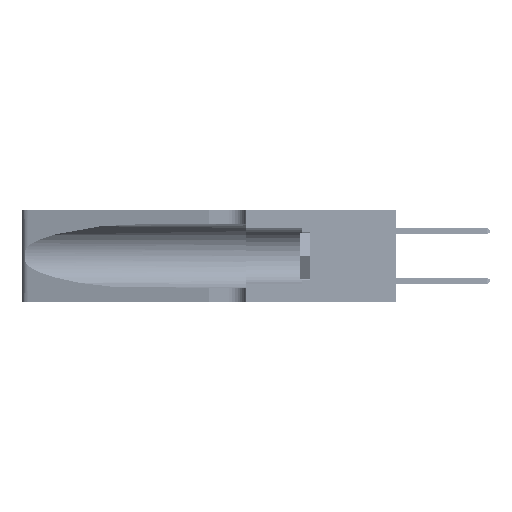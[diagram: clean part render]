
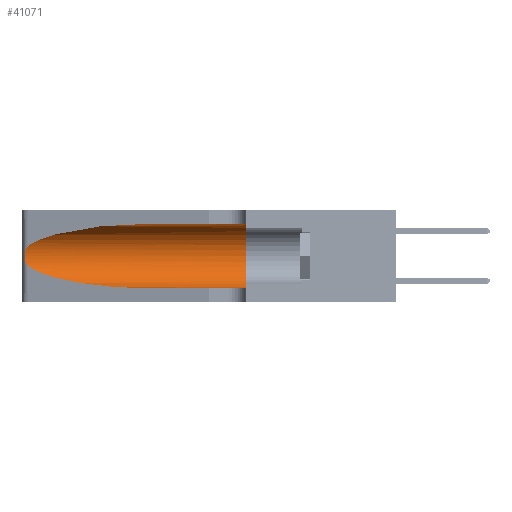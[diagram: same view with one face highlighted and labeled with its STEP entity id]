
A CAD part, left-side view. The second image highlights one B-rep face of the part: STEP entity #41071.
In plain terms, the highlighted cylindrical face has radius 3.308 mm (diameter 6.617 mm), a partial arc.
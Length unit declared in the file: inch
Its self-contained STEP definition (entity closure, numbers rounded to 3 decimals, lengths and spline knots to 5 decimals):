
#475 = CARTESIAN_POINT ( 'NONE',  ( 0.26075, 1.23896, 0.178 ) ) ;
#2468 = ORIENTED_EDGE ( 'NONE', *, *, #50630, .T. ) ;
#2620 = VERTEX_POINT ( 'NONE', #48003 ) ;
#3009 = VERTEX_POINT ( 'NONE', #33559 ) ;
#3518 = B_SPLINE_CURVE_WITH_KNOTS ( 'NONE', 3,
 ( #17410, #34336, #17591, #46937, #21864, #51092, #26085, #475, #30305, #4786, #34519, #9131, #38714, #13441 ),
 .UNSPECIFIED., .F., .F.,
 ( 4, 2, 2, 2, 2, 2, 4 ),
 ( 0., 0.00027, 0.00053, 0.00107, 0.0016, 0.00187, 0.00214 ),
 .UNSPECIFIED. ) ;
#4345 = CARTESIAN_POINT ( 'NONE',  ( 0.1305, 0.35, 0.05475 ) ) ;
#4786 = CARTESIAN_POINT ( 'NONE',  ( 0.25856, 1.23593, 0.16098 ) ) ;
#9131 = CARTESIAN_POINT ( 'NONE',  ( 0.25639, 1.23186, 0.15144 ) ) ;
#10163 = CARTESIAN_POINT ( 'NONE',  ( 0.1305, 1.61858, 0.05475 ) ) ;
#11544 = CARTESIAN_POINT ( 'NONE',  ( 0.1305, 0.72297, 0.05475 ) ) ;
#11662 = LINE ( 'NONE', #10163, #32867 ) ;
#12039 = ORIENTED_EDGE ( 'NONE', *, *, #29531, .T. ) ;
#12723 = CARTESIAN_POINT ( 'NONE',  ( 0.2373, 1.15595, 0.28018 ) ) ;
#13364 = DIRECTION ( 'NONE',  ( 0., 1., 0. ) ) ;
#13441 = CARTESIAN_POINT ( 'NONE',  ( 0.25487, 1.22718, 0.14631 ) ) ;
#14052 = VERTEX_POINT ( 'NONE', #42534 ) ;
#15527 = CARTESIAN_POINT ( 'NONE',  ( 0.1305, 1.61858, 0.31525 ) ) ;
#17410 = CARTESIAN_POINT ( 'NONE',  ( 0.25487, 1.22718, 0.22369 ) ) ;
#17522 = LINE ( 'NONE', #15527, #53520 ) ;
#17591 = CARTESIAN_POINT ( 'NONE',  ( 0.25639, 1.23184, 0.21858 ) ) ;
#18605 = FACE_OUTER_BOUND ( 'NONE', #50829, .T. ) ;
#18633 = CARTESIAN_POINT ( 'NONE',  ( 0.1305, 0.35, 0.31525 ) ) ;
#19845 = ORIENTED_EDGE ( 'NONE', *, *, #38909, .F. ) ;
#20192 = VERTEX_POINT ( 'NONE', #18633 ) ;
#20394 = DIRECTION ( 'NONE',  ( 0., 0., -1. ) ) ;
#20516 = CIRCLE ( 'NONE', #45931, 0.13025 ) ;
#21864 = CARTESIAN_POINT ( 'NONE',  ( 0.25854, 1.2359, 0.20912 ) ) ;
#22410 = EDGE_CURVE ( 'NONE', #14052, #3009, #23417, .T. ) ;
#22873 = DIRECTION ( 'NONE',  ( 0., -1., 0. ) ) ;
#23357 = ORIENTED_EDGE ( 'NONE', *, *, #22410, .T. ) ;
#23417 =( BOUNDED_CURVE ( )  B_SPLINE_CURVE ( 3, ( #54585, #25383, #12723, #42224 ),
 .UNSPECIFIED., .F., .T. ) 
 B_SPLINE_CURVE_WITH_KNOTS ( ( 4, 4 ),
 ( 1.5708, 2.84003 ),
 .UNSPECIFIED. ) 
 CURVE ( )  GEOMETRIC_REPRESENTATION_ITEM ( )  RATIONAL_B_SPLINE_CURVE ( ( 1., 0.87, 0.87, 1. ) ) 
 REPRESENTATION_ITEM ( '' )  );
#24610 = CARTESIAN_POINT ( 'NONE',  ( 0.1305, 1.61858, 0.185 ) ) ;
#25011 = AXIS2_PLACEMENT_3D ( 'NONE', #24610, #53798, #20394 ) ;
#25383 = CARTESIAN_POINT ( 'NONE',  ( 0.18966, 0.96281, 0.31525 ) ) ;
#26085 = CARTESIAN_POINT ( 'NONE',  ( 0.26075, 1.23896, 0.19203 ) ) ;
#29531 = EDGE_CURVE ( 'NONE', #3009, #2620, #3518, .T. ) ;
#29814 = ORIENTED_EDGE ( 'NONE', *, *, #35587, .T. ) ;
#30305 = CARTESIAN_POINT ( 'NONE',  ( 0.26017, 1.23833, 0.17102 ) ) ;
#32675 = CARTESIAN_POINT ( 'NONE',  ( 0.2373, 1.15595, 0.08982 ) ) ;
#32867 = VECTOR ( 'NONE', #22873, 39.37008 ) ;
#33559 = CARTESIAN_POINT ( 'NONE',  ( 0.25487, 1.22718, 0.22369 ) ) ;
#34336 = CARTESIAN_POINT ( 'NONE',  ( 0.25555, 1.22994, 0.2215 ) ) ;
#34519 = CARTESIAN_POINT ( 'NONE',  ( 0.25789, 1.23486, 0.15765 ) ) ;
#34765 = ORIENTED_EDGE ( 'NONE', *, *, #37085, .F. ) ;
#35587 = EDGE_CURVE ( 'NONE', #2620, #45388, #48551, .T. ) ;
#36704 = CARTESIAN_POINT ( 'NONE',  ( 0.25487, 1.22718, 0.14631 ) ) ;
#36880 = CARTESIAN_POINT ( 'NONE',  ( 0.18966, 0.96281, 0.05475 ) ) ;
#37085 = EDGE_CURVE ( 'NONE', #20192, #50388, #20516, .T. ) ;
#38648 = CARTESIAN_POINT ( 'NONE',  ( 0.1305, 0.35, 0.185 ) ) ;
#38714 = CARTESIAN_POINT ( 'NONE',  ( 0.25555, 1.22993, 0.14849 ) ) ;
#38909 = EDGE_CURVE ( 'NONE', #14052, #20192, #17522, .T. ) ;
#39633 = CYLINDRICAL_SURFACE ( 'NONE', #25011, 0.13025 ) ;
#41071 = ADVANCED_FACE ( 'NONE', ( #18605 ), #39633, .F. ) ;
#42224 = CARTESIAN_POINT ( 'NONE',  ( 0.25487, 1.22718, 0.22369 ) ) ;
#42534 = CARTESIAN_POINT ( 'NONE',  ( 0.1305, 0.72297, 0.31525 ) ) ;
#42849 = DIRECTION ( 'NONE',  ( 0., 0., 1. ) ) ;
#44954 = DIRECTION ( 'NONE',  ( 0., -1., 0. ) ) ;
#45388 = VERTEX_POINT ( 'NONE', #54355 ) ;
#45931 = AXIS2_PLACEMENT_3D ( 'NONE', #38648, #13364, #42849 ) ;
#46937 = CARTESIAN_POINT ( 'NONE',  ( 0.25787, 1.23484, 0.2124 ) ) ;
#48003 = CARTESIAN_POINT ( 'NONE',  ( 0.25487, 1.22718, 0.14631 ) ) ;
#48551 =( BOUNDED_CURVE ( )  B_SPLINE_CURVE ( 3, ( #36704, #32675, #36880, #11544 ),
 .UNSPECIFIED., .F., .F. ) 
 B_SPLINE_CURVE_WITH_KNOTS ( ( 4, 4 ),
 ( 3.44316, 4.71239 ),
 .UNSPECIFIED. ) 
 CURVE ( )  GEOMETRIC_REPRESENTATION_ITEM ( )  RATIONAL_B_SPLINE_CURVE ( ( 1., 0.87, 0.87, 1. ) ) 
 REPRESENTATION_ITEM ( '' )  );
#50388 = VERTEX_POINT ( 'NONE', #4345 ) ;
#50630 = EDGE_CURVE ( 'NONE', #45388, #50388, #11662, .T. ) ;
#50829 = EDGE_LOOP ( 'NONE', ( #23357, #12039, #29814, #2468, #34765, #19845 ) ) ;
#51092 = CARTESIAN_POINT ( 'NONE',  ( 0.26018, 1.23835, 0.19895 ) ) ;
#53520 = VECTOR ( 'NONE', #44954, 39.37008 ) ;
#53798 = DIRECTION ( 'NONE',  ( 0., -1., 0. ) ) ;
#54355 = CARTESIAN_POINT ( 'NONE',  ( 0.1305, 0.72297, 0.05475 ) ) ;
#54585 = CARTESIAN_POINT ( 'NONE',  ( 0.1305, 0.72297, 0.31525 ) ) ;
